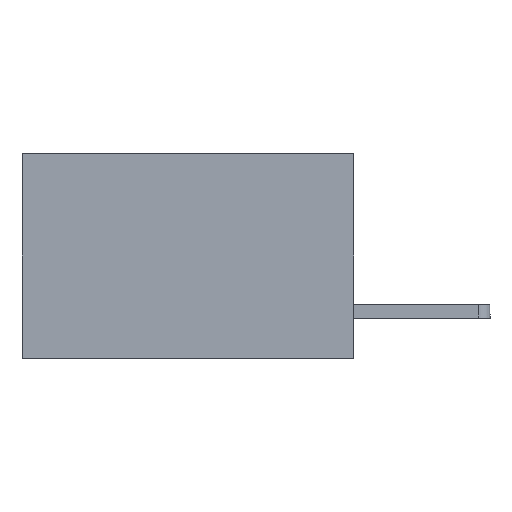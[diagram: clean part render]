
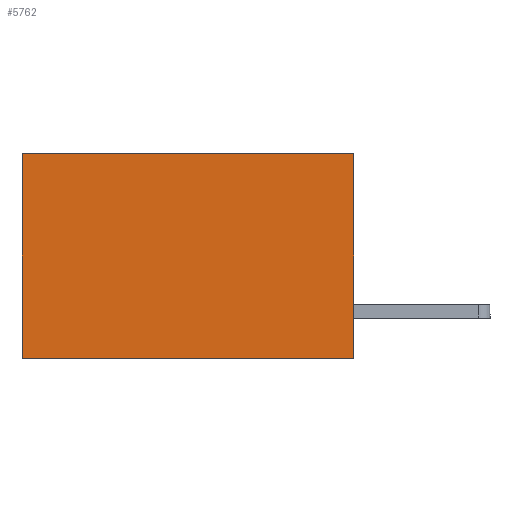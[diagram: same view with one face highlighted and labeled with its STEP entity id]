
A CAD part, left-side view. The second image highlights one B-rep face of the part: STEP entity #5762.
In plain terms, the highlighted planar face has unit normal (-1, 0, 0).
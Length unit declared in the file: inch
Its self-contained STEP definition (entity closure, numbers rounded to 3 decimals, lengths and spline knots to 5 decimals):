
#472 = DIRECTION ( 'NONE',  ( 1., 0., 0. ) ) ;
#1110 = EDGE_LOOP ( 'NONE', ( #7935, #7593, #1267, #3009 ) ) ;
#1267 = ORIENTED_EDGE ( 'NONE', *, *, #2683, .F. ) ;
#1268 = AXIS2_PLACEMENT_3D ( 'NONE', #6304, #472, #5013 ) ;
#1598 = CARTESIAN_POINT ( 'NONE',  ( 0.2875, 0., -0.37 ) ) ;
#1874 = CARTESIAN_POINT ( 'NONE',  ( 0.2875, 0.6, 0. ) ) ;
#1916 = LINE ( 'NONE', #6843, #8406 ) ;
#2410 = PLANE ( 'NONE',  #1268 ) ;
#2683 = EDGE_CURVE ( 'NONE', #5964, #5561, #7942, .T. ) ;
#2809 = CARTESIAN_POINT ( 'NONE',  ( 0.2875, 0., 0. ) ) ;
#2933 = FACE_OUTER_BOUND ( 'NONE', #1110, .T. ) ;
#3009 = ORIENTED_EDGE ( 'NONE', *, *, #4162, .T. ) ;
#4162 = EDGE_CURVE ( 'NONE', #5964, #5857, #1916, .T. ) ;
#4166 = CARTESIAN_POINT ( 'NONE',  ( 0.2875, 0., -0.37 ) ) ;
#4374 = CARTESIAN_POINT ( 'NONE',  ( 0.2875, 0., 0. ) ) ;
#4772 = VERTEX_POINT ( 'NONE', #7374 ) ;
#4983 = DIRECTION ( 'NONE',  ( 0., 0., -1. ) ) ;
#5013 = DIRECTION ( 'NONE',  ( 0., 0., -1. ) ) ;
#5561 = VERTEX_POINT ( 'NONE', #1598 ) ;
#5762 = ADVANCED_FACE ( 'NONE', ( #2933 ), #2410, .F. ) ;
#5857 = VERTEX_POINT ( 'NONE', #1874 ) ;
#5964 = VERTEX_POINT ( 'NONE', #4374 ) ;
#6304 = CARTESIAN_POINT ( 'NONE',  ( 0.2875, 0., 0. ) ) ;
#6460 = VECTOR ( 'NONE', #4983, 39.37008 ) ;
#6788 = EDGE_CURVE ( 'NONE', #5561, #4772, #6862, .T. ) ;
#6824 = EDGE_CURVE ( 'NONE', #5857, #4772, #8179, .T. ) ;
#6843 = CARTESIAN_POINT ( 'NONE',  ( 0.2875, 0., 0. ) ) ;
#6862 = LINE ( 'NONE', #4166, #8378 ) ;
#6875 = DIRECTION ( 'NONE',  ( 0., 1., 0. ) ) ;
#7357 = DIRECTION ( 'NONE',  ( 0., 0., -1. ) ) ;
#7374 = CARTESIAN_POINT ( 'NONE',  ( 0.2875, 0.6, -0.37 ) ) ;
#7569 = CARTESIAN_POINT ( 'NONE',  ( 0.2875, 0.6, 0. ) ) ;
#7593 = ORIENTED_EDGE ( 'NONE', *, *, #6788, .F. ) ;
#7935 = ORIENTED_EDGE ( 'NONE', *, *, #6824, .T. ) ;
#7942 = LINE ( 'NONE', #2809, #8150 ) ;
#8150 = VECTOR ( 'NONE', #7357, 39.37008 ) ;
#8156 = DIRECTION ( 'NONE',  ( 0., 1., 0. ) ) ;
#8179 = LINE ( 'NONE', #7569, #6460 ) ;
#8378 = VECTOR ( 'NONE', #6875, 39.37008 ) ;
#8406 = VECTOR ( 'NONE', #8156, 39.37008 ) ;
